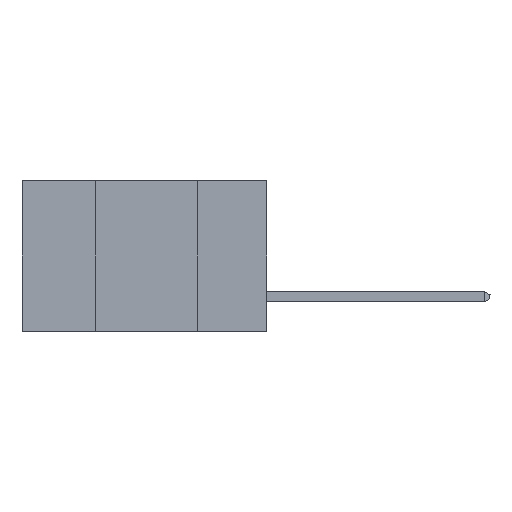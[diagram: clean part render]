
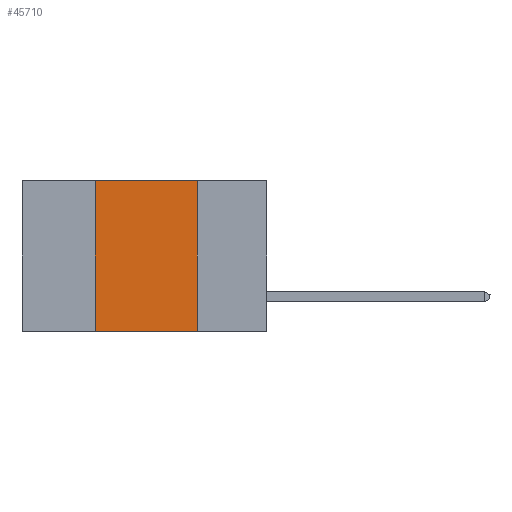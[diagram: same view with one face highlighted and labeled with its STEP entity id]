
A CAD part, left-side view. The second image highlights one B-rep face of the part: STEP entity #45710.
In plain terms, the highlighted planar face has unit normal (-1, 0, 0).
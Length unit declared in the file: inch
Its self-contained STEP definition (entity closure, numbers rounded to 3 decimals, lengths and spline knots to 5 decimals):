
#207 = CARTESIAN_POINT ( 'NONE',  ( 0., 0.42, 0. ) ) ;
#394 = VERTEX_POINT ( 'NONE', #39495 ) ;
#563 = VECTOR ( 'NONE', #22937, 39.37008 ) ;
#2082 = DIRECTION ( 'NONE',  ( 0., 0., -1. ) ) ;
#3923 = DIRECTION ( 'NONE',  ( 0., 0., 1. ) ) ;
#10383 = LINE ( 'NONE', #41149, #563 ) ;
#10686 = DIRECTION ( 'NONE',  ( 0., -1., 0. ) ) ;
#11832 = CARTESIAN_POINT ( 'NONE',  ( 0., 0.17, -0.37 ) ) ;
#14685 = VERTEX_POINT ( 'NONE', #11832 ) ;
#15266 = DIRECTION ( 'NONE',  ( 0., 0., -1. ) ) ;
#16599 = VECTOR ( 'NONE', #3923, 39.37008 ) ;
#19269 = CARTESIAN_POINT ( 'NONE',  ( 0., 0.6, 0. ) ) ;
#20385 = ORIENTED_EDGE ( 'NONE', *, *, #39197, .F. ) ;
#22937 = DIRECTION ( 'NONE',  ( 0., -1., 0. ) ) ;
#24038 = EDGE_CURVE ( 'NONE', #394, #24371, #10383, .T. ) ;
#24108 = CARTESIAN_POINT ( 'NONE',  ( 0., 0.17, 0. ) ) ;
#24371 = VERTEX_POINT ( 'NONE', #46473 ) ;
#27306 = ORIENTED_EDGE ( 'NONE', *, *, #28855, .T. ) ;
#28855 = EDGE_CURVE ( 'NONE', #29069, #14685, #44361, .T. ) ;
#29069 = VERTEX_POINT ( 'NONE', #30639 ) ;
#29662 = EDGE_CURVE ( 'NONE', #29069, #394, #36195, .T. ) ;
#30639 = CARTESIAN_POINT ( 'NONE',  ( 0., 0.42, -0.37 ) ) ;
#34076 = FACE_OUTER_BOUND ( 'NONE', #45164, .T. ) ;
#36195 = LINE ( 'NONE', #207, #16599 ) ;
#37248 = VECTOR ( 'NONE', #2082, 39.37008 ) ;
#37502 = DIRECTION ( 'NONE',  ( 1., 0., 0. ) ) ;
#37669 = PLANE ( 'NONE',  #39047 ) ;
#37810 = ORIENTED_EDGE ( 'NONE', *, *, #29662, .F. ) ;
#38421 = LINE ( 'NONE', #24108, #37248 ) ;
#39047 = AXIS2_PLACEMENT_3D ( 'NONE', #19269, #37502, #15266 ) ;
#39197 = EDGE_CURVE ( 'NONE', #24371, #14685, #38421, .T. ) ;
#39495 = CARTESIAN_POINT ( 'NONE',  ( 0., 0.42, 0. ) ) ;
#39811 = ORIENTED_EDGE ( 'NONE', *, *, #24038, .F. ) ;
#40654 = CARTESIAN_POINT ( 'NONE',  ( 0., 0.6, -0.37 ) ) ;
#40877 = VECTOR ( 'NONE', #10686, 39.37008 ) ;
#41149 = CARTESIAN_POINT ( 'NONE',  ( 0., 0.6, 0. ) ) ;
#44361 = LINE ( 'NONE', #40654, #40877 ) ;
#45164 = EDGE_LOOP ( 'NONE', ( #20385, #39811, #37810, #27306 ) ) ;
#45710 = ADVANCED_FACE ( 'NONE', ( #34076 ), #37669, .F. ) ;
#46473 = CARTESIAN_POINT ( 'NONE',  ( 0., 0.17, 0. ) ) ;
